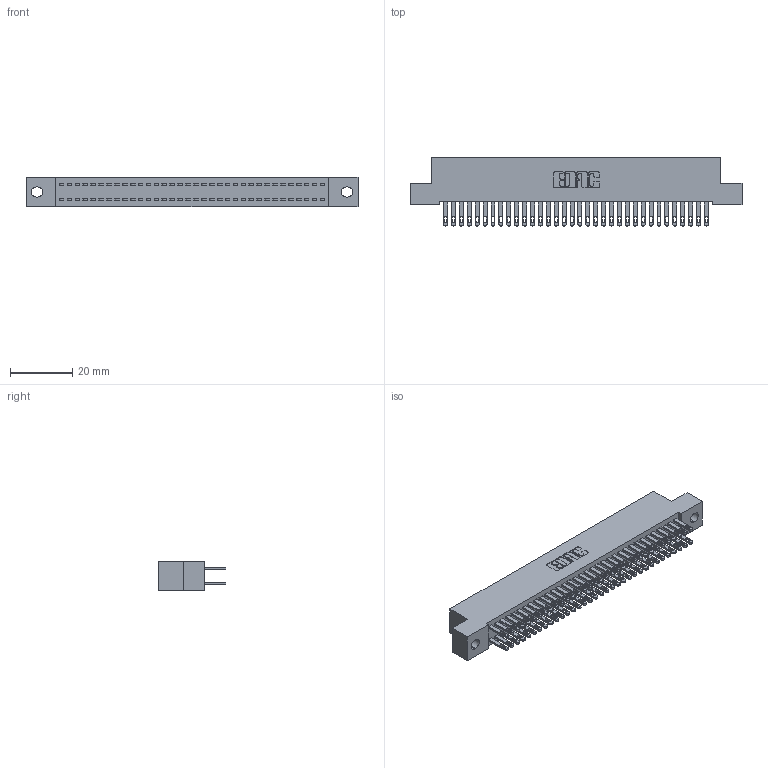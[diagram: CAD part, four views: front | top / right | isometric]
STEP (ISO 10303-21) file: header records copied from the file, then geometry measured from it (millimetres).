
FILE_DESCRIPTION (( 'STEP AP203' ), '1' );
FILE_NAME ('342-068-500-202.STEP', '2019-10-03T15:14:42', ( '' ), ( '' ), 'SwSTEP 2.0', 'SolidWorks 2016', '' );
FILE_SCHEMA (( 'CONFIG_CONTROL_DESIGN' ));
Length unit declared in the file: inch
Products named in the file (3): 342 Part_.128 Slot; 345-292-001_345-293-100; 342-068-500-202
Assembly tree (69 placements, depth 2):
  342-068-500-202
    342 Part_.128 Slot
    345-292-001_345-293-100  x68
Bounding box: 106.68 x 21.85 x 9.4 mm (x, y, z)
Volume: 9703 mm3; surface area: 16007.4 mm2
Topology: 69 solids, 69 shells, 3378 faces, 10307 edges, 6870 vertices
Faces by surface type: plane 2110, cylinder 1268
Entity records: 22841 total; most frequent: CARTESIAN_POINT 3794, ORIENTED_EDGE 3730, DIRECTION 3257, EDGE_CURVE 1865, VECTOR 1733, LINE 1733, VERTEX_POINT 1242, AXIS2_PLACEMENT_3D 762
